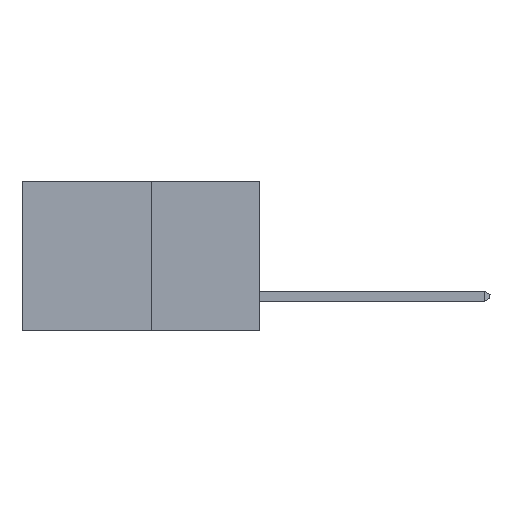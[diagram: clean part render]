
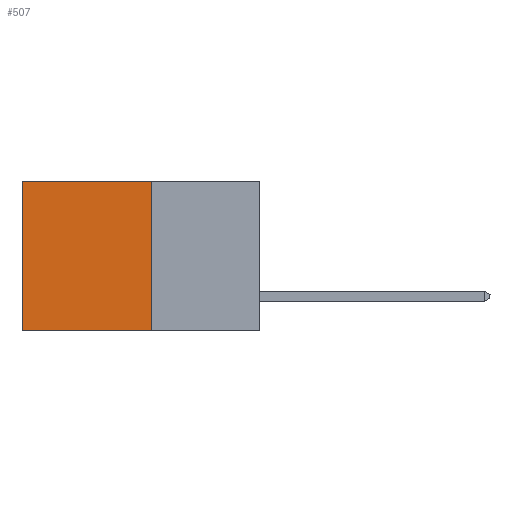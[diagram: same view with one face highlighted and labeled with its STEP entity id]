
A CAD part, left-side view. The second image highlights one B-rep face of the part: STEP entity #507.
In plain terms, the highlighted planar face has unit normal (-1, 0, 0).
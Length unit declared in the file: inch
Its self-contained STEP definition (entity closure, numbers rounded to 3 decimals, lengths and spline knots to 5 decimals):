
#345 = LINE ( 'NONE', #7628, #623 ) ;
#475 = ORIENTED_EDGE ( 'NONE', *, *, #11056, .T. ) ;
#507 = ADVANCED_FACE ( 'NONE', ( #6541 ), #4176, .F. ) ;
#623 = VECTOR ( 'NONE', #9273, 39.37008 ) ;
#975 = CARTESIAN_POINT ( 'NONE',  ( 0.277, 0.27, -0.37 ) ) ;
#1329 = LINE ( 'NONE', #5369, #8080 ) ;
#1639 = CARTESIAN_POINT ( 'NONE',  ( 0.277, 0.27, 0. ) ) ;
#1909 = VERTEX_POINT ( 'NONE', #1639 ) ;
#2141 = VERTEX_POINT ( 'NONE', #4097 ) ;
#2263 = EDGE_CURVE ( 'NONE', #11043, #4750, #1329, .T. ) ;
#4097 = CARTESIAN_POINT ( 'NONE',  ( 0.277, 0.59, 0. ) ) ;
#4176 = PLANE ( 'NONE',  #8368 ) ;
#4635 = EDGE_CURVE ( 'NONE', #1909, #11043, #345, .T. ) ;
#4636 = CARTESIAN_POINT ( 'NONE',  ( 0.277, 0.27, 0. ) ) ;
#4750 = VERTEX_POINT ( 'NONE', #7101 ) ;
#4921 = ORIENTED_EDGE ( 'NONE', *, *, #4635, .F. ) ;
#5077 = DIRECTION ( 'NONE',  ( 1., 0., 0. ) ) ;
#5313 = EDGE_LOOP ( 'NONE', ( #9122, #9598, #4921, #475 ) ) ;
#5362 = CARTESIAN_POINT ( 'NONE',  ( 0.277, 0.27, -0.37 ) ) ;
#5369 = CARTESIAN_POINT ( 'NONE',  ( 0.277, 0.27, -0.37 ) ) ;
#6073 = CARTESIAN_POINT ( 'NONE',  ( 0.277, 0.59, -0.37 ) ) ;
#6187 = LINE ( 'NONE', #6073, #10357 ) ;
#6502 = DIRECTION ( 'NONE',  ( 0., 0., -1. ) ) ;
#6541 = FACE_OUTER_BOUND ( 'NONE', #5313, .T. ) ;
#7101 = CARTESIAN_POINT ( 'NONE',  ( 0.277, 0.59, -0.37 ) ) ;
#7474 = EDGE_CURVE ( 'NONE', #2141, #4750, #6187, .T. ) ;
#7584 = DIRECTION ( 'NONE',  ( 0., 1., 0. ) ) ;
#7628 = CARTESIAN_POINT ( 'NONE',  ( 0.277, 0.27, -0.37 ) ) ;
#8080 = VECTOR ( 'NONE', #7584, 39.37008 ) ;
#8255 = VECTOR ( 'NONE', #10522, 39.37008 ) ;
#8368 = AXIS2_PLACEMENT_3D ( 'NONE', #5362, #5077, #6502 ) ;
#9122 = ORIENTED_EDGE ( 'NONE', *, *, #7474, .T. ) ;
#9273 = DIRECTION ( 'NONE',  ( 0., 0., -1. ) ) ;
#9598 = ORIENTED_EDGE ( 'NONE', *, *, #2263, .F. ) ;
#10209 = LINE ( 'NONE', #4636, #8255 ) ;
#10357 = VECTOR ( 'NONE', #11029, 39.37008 ) ;
#10522 = DIRECTION ( 'NONE',  ( 0., 1., 0. ) ) ;
#11029 = DIRECTION ( 'NONE',  ( 0., 0., -1. ) ) ;
#11043 = VERTEX_POINT ( 'NONE', #975 ) ;
#11056 = EDGE_CURVE ( 'NONE', #1909, #2141, #10209, .T. ) ;
